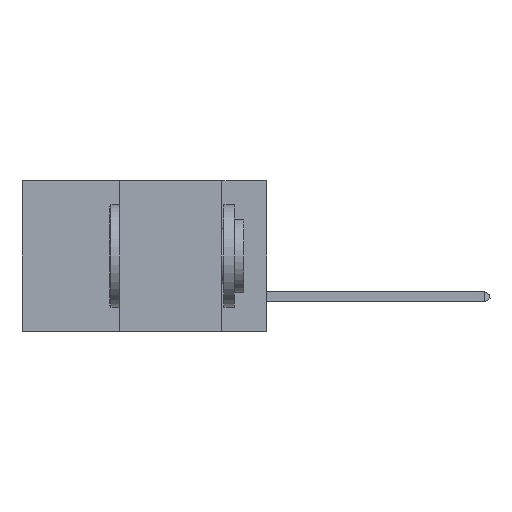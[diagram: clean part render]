
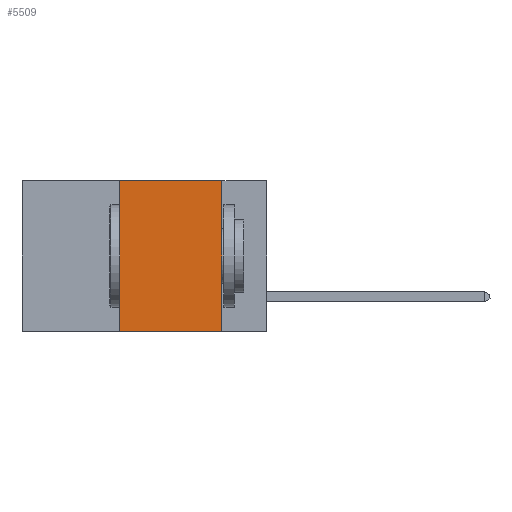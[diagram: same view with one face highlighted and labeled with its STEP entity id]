
A CAD part, left-side view. The second image highlights one B-rep face of the part: STEP entity #5509.
In plain terms, the highlighted planar face has unit normal (-1, 0, 0).
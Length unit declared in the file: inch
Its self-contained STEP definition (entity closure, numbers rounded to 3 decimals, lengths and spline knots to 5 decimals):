
#1488 = VECTOR ( 'NONE', #43417, 39.37008 ) ;
#1600 = ORIENTED_EDGE ( 'NONE', *, *, #22385, .F. ) ;
#2090 = DIRECTION ( 'NONE',  ( 1., 0., 0. ) ) ;
#2379 = DIRECTION ( 'NONE',  ( 0., 0., -1. ) ) ;
#3023 = VERTEX_POINT ( 'NONE', #10570 ) ;
#5509 = ADVANCED_FACE ( 'NONE', ( #17536 ), #22556, .F. ) ;
#5969 = ORIENTED_EDGE ( 'NONE', *, *, #39509, .F. ) ;
#6744 = DIRECTION ( 'NONE',  ( 0., -1., 0. ) ) ;
#10570 = CARTESIAN_POINT ( 'NONE',  ( 0., 0.36, -0.37 ) ) ;
#11390 = CARTESIAN_POINT ( 'NONE',  ( 0., 0.36, 0. ) ) ;
#11489 = VECTOR ( 'NONE', #17295, 39.37008 ) ;
#16950 = LINE ( 'NONE', #37143, #36854 ) ;
#17295 = DIRECTION ( 'NONE',  ( 0., -1., 0. ) ) ;
#17536 = FACE_OUTER_BOUND ( 'NONE', #39372, .T. ) ;
#17747 = CARTESIAN_POINT ( 'NONE',  ( 0., 0.6, 0. ) ) ;
#20154 = VECTOR ( 'NONE', #28600, 39.37008 ) ;
#21027 = LINE ( 'NONE', #17747, #11489 ) ;
#22385 = EDGE_CURVE ( 'NONE', #3023, #28587, #41640, .T. ) ;
#22556 = PLANE ( 'NONE',  #33765 ) ;
#22713 = VERTEX_POINT ( 'NONE', #37283 ) ;
#22736 = EDGE_CURVE ( 'NONE', #3023, #22713, #16950, .T. ) ;
#26448 = CARTESIAN_POINT ( 'NONE',  ( 0., 0.11, 0. ) ) ;
#27707 = CARTESIAN_POINT ( 'NONE',  ( 0., 0.11, 0. ) ) ;
#28329 = EDGE_CURVE ( 'NONE', #29057, #22713, #33580, .T. ) ;
#28587 = VERTEX_POINT ( 'NONE', #11390 ) ;
#28600 = DIRECTION ( 'NONE',  ( 0., 0., 1. ) ) ;
#29057 = VERTEX_POINT ( 'NONE', #27707 ) ;
#29317 = CARTESIAN_POINT ( 'NONE',  ( 0., 0.6, 0. ) ) ;
#33580 = LINE ( 'NONE', #26448, #1488 ) ;
#33765 = AXIS2_PLACEMENT_3D ( 'NONE', #29317, #2090, #2379 ) ;
#36854 = VECTOR ( 'NONE', #6744, 39.37008 ) ;
#37143 = CARTESIAN_POINT ( 'NONE',  ( 0., 0.6, -0.37 ) ) ;
#37283 = CARTESIAN_POINT ( 'NONE',  ( 0., 0.11, -0.37 ) ) ;
#38146 = ORIENTED_EDGE ( 'NONE', *, *, #28329, .F. ) ;
#39372 = EDGE_LOOP ( 'NONE', ( #38146, #5969, #1600, #41052 ) ) ;
#39509 = EDGE_CURVE ( 'NONE', #28587, #29057, #21027, .T. ) ;
#41052 = ORIENTED_EDGE ( 'NONE', *, *, #22736, .T. ) ;
#41640 = LINE ( 'NONE', #41882, #20154 ) ;
#41882 = CARTESIAN_POINT ( 'NONE',  ( 0., 0.36, 0. ) ) ;
#43417 = DIRECTION ( 'NONE',  ( 0., 0., -1. ) ) ;
